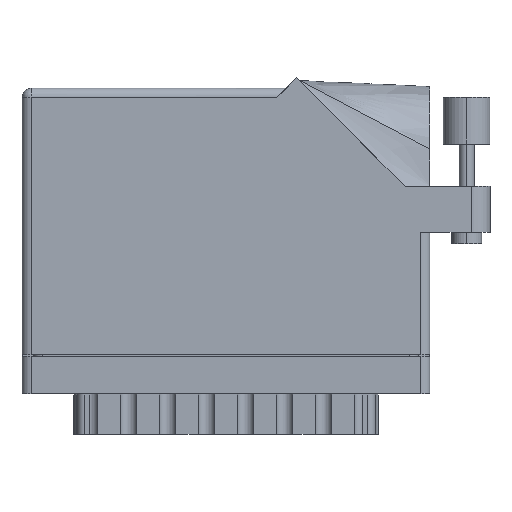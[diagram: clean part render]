
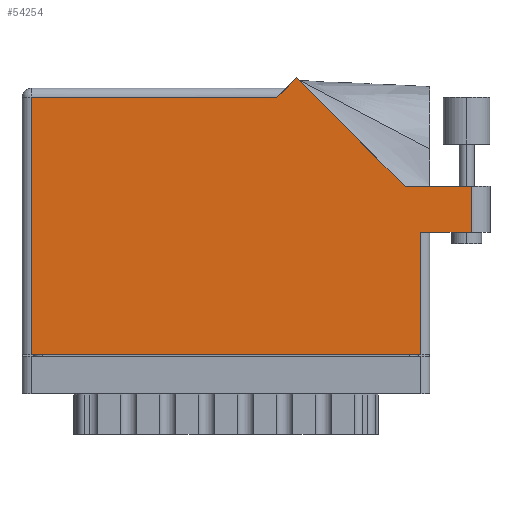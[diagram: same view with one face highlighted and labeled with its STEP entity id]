
A CAD part, front view. The second image highlights one B-rep face of the part: STEP entity #54254.
In plain terms, the highlighted face is planar.
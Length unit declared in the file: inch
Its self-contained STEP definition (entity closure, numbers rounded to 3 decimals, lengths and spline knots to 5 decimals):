
#129 = CARTESIAN_POINT ( 'NONE',  ( 3.118, 1.122, 0. ) ) ;
#237 = CARTESIAN_POINT ( 'NONE',  ( 0., 1.775, 0. ) ) ;
#286 = DIRECTION ( 'NONE',  ( 1., 0., 0. ) ) ;
#1729 = ORIENTED_EDGE ( 'NONE', *, *, #28961, .T. ) ;
#1998 = AXIS2_PLACEMENT_3D ( 'NONE', #237, #40863, #51152 ) ;
#2037 = DIRECTION ( 'NONE',  ( 0., 1., 0. ) ) ;
#3343 = VERTEX_POINT ( 'NONE', #37495 ) ;
#4479 = VERTEX_POINT ( 'NONE', #16687 ) ;
#4485 = CARTESIAN_POINT ( 'NONE',  ( 2.656, 0.815, 0. ) ) ;
#4787 = DIRECTION ( 'NONE',  ( -1., 0., 0. ) ) ;
#5405 = DIRECTION ( 'NONE',  ( -0.707, -0.707, 0. ) ) ;
#6034 = EDGE_CURVE ( 'NONE', #53073, #51289, #24400, .T. ) ;
#7260 = VERTEX_POINT ( 'NONE', #27608 ) ;
#7626 = EDGE_CURVE ( 'NONE', #40132, #3343, #50416, .T. ) ;
#9578 = DIRECTION ( 'NONE',  ( 0., 1., 0. ) ) ;
#10187 = CARTESIAN_POINT ( 'NONE',  ( 0.062, 0., 0. ) ) ;
#10862 = CARTESIAN_POINT ( 'NONE',  ( 2.993, 1.122, 0. ) ) ;
#11804 = CARTESIAN_POINT ( 'NONE',  ( 0.062, 0., 0. ) ) ;
#13135 = ORIENTED_EDGE ( 'NONE', *, *, #49489, .T. ) ;
#13458 = LINE ( 'NONE', #19776, #15084 ) ;
#13884 = PLANE ( 'NONE',  #1998 ) ;
#14635 = VECTOR ( 'NONE', #2037, 39.37008 ) ;
#15084 = VECTOR ( 'NONE', #9578, 39.37008 ) ;
#15639 = CARTESIAN_POINT ( 'NONE',  ( 1.758, 1.775, 0. ) ) ;
#15709 = CARTESIAN_POINT ( 'NONE',  ( 0., 0., 0. ) ) ;
#16687 = CARTESIAN_POINT ( 'NONE',  ( 1.696, 1.713, 0. ) ) ;
#19407 = ORIENTED_EDGE ( 'NONE', *, *, #64472, .T. ) ;
#19776 = CARTESIAN_POINT ( 'NONE',  ( 2.656, 0.815, 0. ) ) ;
#20751 = DIRECTION ( 'NONE',  ( -1., 0., 0. ) ) ;
#21151 = VECTOR ( 'NONE', #30985, 39.37008 ) ;
#21219 = EDGE_CURVE ( 'NONE', #23117, #40132, #51728, .T. ) ;
#22939 = EDGE_CURVE ( 'NONE', #63233, #65789, #55515, .T. ) ;
#23117 = VERTEX_POINT ( 'NONE', #10862 ) ;
#24400 = LINE ( 'NONE', #62387, #21151 ) ;
#25110 = CARTESIAN_POINT ( 'NONE',  ( 0.062, 1.713, 0. ) ) ;
#27608 = CARTESIAN_POINT ( 'NONE',  ( 2.656, 0., 0. ) ) ;
#28391 = VECTOR ( 'NONE', #58316, 39.37008 ) ;
#28438 = LINE ( 'NONE', #15639, #39775 ) ;
#28961 = EDGE_CURVE ( 'NONE', #4479, #63233, #64460, .T. ) ;
#29004 = ORIENTED_EDGE ( 'NONE', *, *, #22939, .T. ) ;
#29429 = FACE_OUTER_BOUND ( 'NONE', #47661, .T. ) ;
#30254 = CARTESIAN_POINT ( 'NONE',  ( 0., 1.713, 0. ) ) ;
#30985 = DIRECTION ( 'NONE',  ( 1., 0., 0. ) ) ;
#33352 = LINE ( 'NONE', #15709, #61898 ) ;
#34265 = EDGE_CURVE ( 'NONE', #51289, #23117, #56172, .T. ) ;
#37495 = CARTESIAN_POINT ( 'NONE',  ( 1.82871, 1.84571, 0. ) ) ;
#39775 = VECTOR ( 'NONE', #5405, 39.37008 ) ;
#40016 = ORIENTED_EDGE ( 'NONE', *, *, #6034, .T. ) ;
#40132 = VERTEX_POINT ( 'NONE', #49920 ) ;
#40863 = DIRECTION ( 'NONE',  ( 0., 0., -1. ) ) ;
#41760 = EDGE_CURVE ( 'NONE', #7260, #53073, #13458, .T. ) ;
#42269 = CARTESIAN_POINT ( 'NONE',  ( 2.993, 0.815, 0. ) ) ;
#43491 = VECTOR ( 'NONE', #20751, 39.37008 ) ;
#44578 = ORIENTED_EDGE ( 'NONE', *, *, #21219, .T. ) ;
#44844 = VECTOR ( 'NONE', #66809, 39.37008 ) ;
#44888 = VECTOR ( 'NONE', #4787, 39.37008 ) ;
#47661 = EDGE_LOOP ( 'NONE', ( #40016, #60380, #44578, #65282, #19407, #1729, #29004, #13135, #58825 ) ) ;
#49489 = EDGE_CURVE ( 'NONE', #65789, #7260, #33352, .T. ) ;
#49920 = CARTESIAN_POINT ( 'NONE',  ( 2.55242, 1.122, 0. ) ) ;
#50416 = LINE ( 'NONE', #57625, #28391 ) ;
#51152 = DIRECTION ( 'NONE',  ( -1., 0., 0. ) ) ;
#51289 = VERTEX_POINT ( 'NONE', #42269 ) ;
#51728 = LINE ( 'NONE', #129, #43491 ) ;
#53073 = VERTEX_POINT ( 'NONE', #4485 ) ;
#54254 = ADVANCED_FACE ( 'NONE', ( #29429 ), #13884, .F. ) ;
#55515 = LINE ( 'NONE', #10187, #44844 ) ;
#56172 = LINE ( 'NONE', #59146, #14635 ) ;
#57625 = CARTESIAN_POINT ( 'NONE',  ( 2.55242, 1.122, 0. ) ) ;
#58316 = DIRECTION ( 'NONE',  ( -0.707, 0.707, 0. ) ) ;
#58825 = ORIENTED_EDGE ( 'NONE', *, *, #41760, .T. ) ;
#59146 = CARTESIAN_POINT ( 'NONE',  ( 2.993, 1.122, 0. ) ) ;
#60380 = ORIENTED_EDGE ( 'NONE', *, *, #34265, .T. ) ;
#61898 = VECTOR ( 'NONE', #286, 39.37008 ) ;
#62387 = CARTESIAN_POINT ( 'NONE',  ( 2.718, 0.815, 0. ) ) ;
#63233 = VERTEX_POINT ( 'NONE', #25110 ) ;
#64460 = LINE ( 'NONE', #30254, #44888 ) ;
#64472 = EDGE_CURVE ( 'NONE', #3343, #4479, #28438, .T. ) ;
#65282 = ORIENTED_EDGE ( 'NONE', *, *, #7626, .T. ) ;
#65789 = VERTEX_POINT ( 'NONE', #11804 ) ;
#66809 = DIRECTION ( 'NONE',  ( 0., -1., 0. ) ) ;
